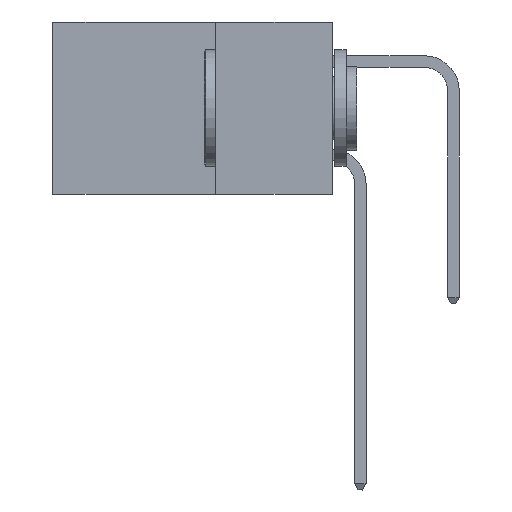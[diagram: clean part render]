
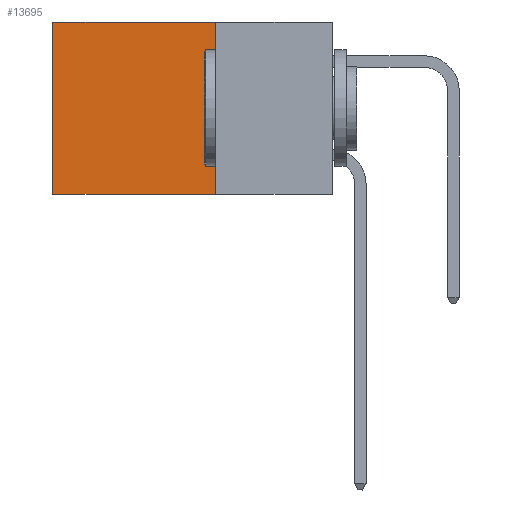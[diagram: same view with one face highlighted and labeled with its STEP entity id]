
A CAD part, left-side view. The second image highlights one B-rep face of the part: STEP entity #13695.
In plain terms, the highlighted planar face has unit normal (-1, 0, 0).
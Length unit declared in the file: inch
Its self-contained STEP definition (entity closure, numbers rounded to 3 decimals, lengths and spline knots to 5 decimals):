
#914 = CARTESIAN_POINT ( 'NONE',  ( 0.298, 0.25, 0. ) ) ;
#2496 = EDGE_CURVE ( 'NONE', #17172, #15841, #9105, .T. ) ;
#2509 = AXIS2_PLACEMENT_3D ( 'NONE', #914, #18660, #5358 ) ;
#3948 = EDGE_CURVE ( 'NONE', #11054, #15841, #18028, .T. ) ;
#5358 = DIRECTION ( 'NONE',  ( 0., 0., -1. ) ) ;
#5559 = ORIENTED_EDGE ( 'NONE', *, *, #8660, .F. ) ;
#5646 = DIRECTION ( 'NONE',  ( 0., 1., 0. ) ) ;
#5874 = CARTESIAN_POINT ( 'NONE',  ( 0.298, 0.25, -0.37 ) ) ;
#6226 = VECTOR ( 'NONE', #21169, 39.37008 ) ;
#6313 = DIRECTION ( 'NONE',  ( 0., 1., 0. ) ) ;
#7433 = CARTESIAN_POINT ( 'NONE',  ( 0.298, 0.25, 0. ) ) ;
#8660 = EDGE_CURVE ( 'NONE', #25600, #17172, #8959, .T. ) ;
#8959 = LINE ( 'NONE', #13352, #14181 ) ;
#9105 = LINE ( 'NONE', #5874, #13618 ) ;
#11054 = VERTEX_POINT ( 'NONE', #24934 ) ;
#11500 = VECTOR ( 'NONE', #6313, 39.37008 ) ;
#12025 = PLANE ( 'NONE',  #2509 ) ;
#13352 = CARTESIAN_POINT ( 'NONE',  ( 0.298, 0.25, 0. ) ) ;
#13606 = ORIENTED_EDGE ( 'NONE', *, *, #18066, .T. ) ;
#13618 = VECTOR ( 'NONE', #5646, 39.37008 ) ;
#13695 = ADVANCED_FACE ( 'NONE', ( #28338 ), #12025, .F. ) ;
#14081 = ORIENTED_EDGE ( 'NONE', *, *, #3948, .T. ) ;
#14181 = VECTOR ( 'NONE', #20006, 39.37008 ) ;
#15841 = VERTEX_POINT ( 'NONE', #20681 ) ;
#16751 = CARTESIAN_POINT ( 'NONE',  ( 0.298, 0.25, -0.37 ) ) ;
#17172 = VERTEX_POINT ( 'NONE', #16751 ) ;
#17334 = LINE ( 'NONE', #21790, #11500 ) ;
#18028 = LINE ( 'NONE', #20967, #6226 ) ;
#18066 = EDGE_CURVE ( 'NONE', #25600, #11054, #17334, .T. ) ;
#18660 = DIRECTION ( 'NONE',  ( 1., 0., 0. ) ) ;
#20006 = DIRECTION ( 'NONE',  ( 0., 0., -1. ) ) ;
#20681 = CARTESIAN_POINT ( 'NONE',  ( 0.298, 0.6, -0.37 ) ) ;
#20967 = CARTESIAN_POINT ( 'NONE',  ( 0.298, 0.6, 0. ) ) ;
#21169 = DIRECTION ( 'NONE',  ( 0., 0., -1. ) ) ;
#21790 = CARTESIAN_POINT ( 'NONE',  ( 0.298, 0.25, 0. ) ) ;
#23103 = ORIENTED_EDGE ( 'NONE', *, *, #2496, .F. ) ;
#23720 = EDGE_LOOP ( 'NONE', ( #14081, #23103, #5559, #13606 ) ) ;
#24934 = CARTESIAN_POINT ( 'NONE',  ( 0.298, 0.6, 0. ) ) ;
#25600 = VERTEX_POINT ( 'NONE', #7433 ) ;
#28338 = FACE_OUTER_BOUND ( 'NONE', #23720, .T. ) ;
